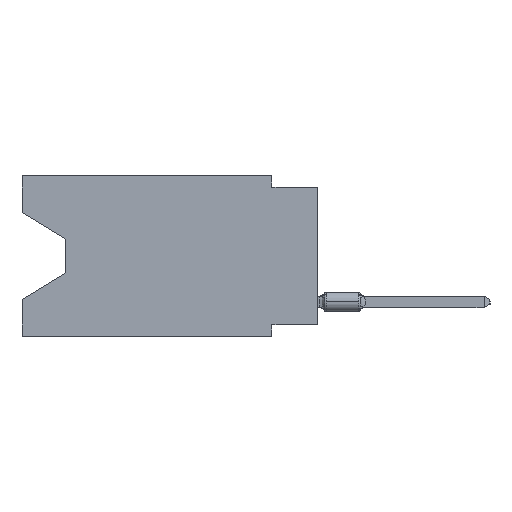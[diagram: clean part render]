
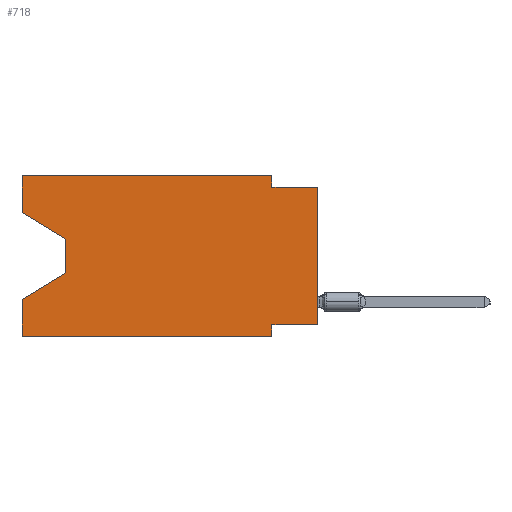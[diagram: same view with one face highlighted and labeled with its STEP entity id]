
A CAD part, left-side view. The second image highlights one B-rep face of the part: STEP entity #718.
In plain terms, the highlighted planar face has unit normal (-1, 0, 0).
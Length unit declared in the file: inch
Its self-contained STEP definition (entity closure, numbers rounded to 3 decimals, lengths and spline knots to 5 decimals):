
#529 = VERTEX_POINT ( 'NONE', #28425 ) ;
#718 = ADVANCED_FACE ( 'NONE', ( #73550 ), #9731, .F. ) ;
#1139 = EDGE_CURVE ( 'NONE', #39890, #15098, #31501, .T. ) ;
#1397 = CARTESIAN_POINT ( 'NONE',  ( 0., 0.55, -0.212 ) ) ;
#1615 = CARTESIAN_POINT ( 'NONE',  ( 0., 0.55, -0.138 ) ) ;
#1846 = VECTOR ( 'NONE', #88715, 39.37008 ) ;
#2038 = CARTESIAN_POINT ( 'NONE',  ( 0., 0.55, -0.138 ) ) ;
#2410 = LINE ( 'NONE', #39551, #10619 ) ;
#2520 = DIRECTION ( 'NONE',  ( 0., 0., -1. ) ) ;
#3393 = ORIENTED_EDGE ( 'NONE', *, *, #14539, .F. ) ;
#3409 = VERTEX_POINT ( 'NONE', #2038 ) ;
#3998 = VECTOR ( 'NONE', #41100, 39.37008 ) ;
#4539 = ORIENTED_EDGE ( 'NONE', *, *, #81420, .F. ) ;
#5720 = EDGE_CURVE ( 'NONE', #39890, #23113, #46511, .T. ) ;
#6797 = VECTOR ( 'NONE', #34415, 39.37008 ) ;
#7557 = ORIENTED_EDGE ( 'NONE', *, *, #41172, .T. ) ;
#9021 = VERTEX_POINT ( 'NONE', #71964 ) ;
#9731 = PLANE ( 'NONE',  #26192 ) ;
#10619 = VECTOR ( 'NONE', #87666, 39.37008 ) ;
#12242 = CARTESIAN_POINT ( 'NONE',  ( 0., 0.1, 0. ) ) ;
#12464 = ORIENTED_EDGE ( 'NONE', *, *, #36770, .F. ) ;
#12671 = LINE ( 'NONE', #49007, #3998 ) ;
#12762 = VERTEX_POINT ( 'NONE', #62096 ) ;
#12783 = EDGE_CURVE ( 'NONE', #80921, #50967, #25815, .T. ) ;
#13829 = VECTOR ( 'NONE', #77037, 39.37008 ) ;
#14100 = VECTOR ( 'NONE', #76528, 39.37008 ) ;
#14539 = EDGE_CURVE ( 'NONE', #50967, #12762, #84427, .T. ) ;
#15098 = VERTEX_POINT ( 'NONE', #60934 ) ;
#17013 = LINE ( 'NONE', #67295, #1846 ) ;
#17425 = CARTESIAN_POINT ( 'NONE',  ( 0., 0.645, 0. ) ) ;
#17996 = CARTESIAN_POINT ( 'NONE',  ( 0., 0.645, -0.35 ) ) ;
#19240 = VECTOR ( 'NONE', #33089, 39.37008 ) ;
#19480 = DIRECTION ( 'NONE',  ( 1., 0., 0. ) ) ;
#19535 = ORIENTED_EDGE ( 'NONE', *, *, #32777, .F. ) ;
#20206 = LINE ( 'NONE', #48613, #13829 ) ;
#22618 = EDGE_CURVE ( 'NONE', #48792, #23113, #12671, .T. ) ;
#23048 = EDGE_LOOP ( 'NONE', ( #25840, #46961, #44289, #46585, #39446, #19535, #4539, #7557, #12464, #3393, #65262, #60566 ) ) ;
#23113 = VERTEX_POINT ( 'NONE', #63306 ) ;
#25268 = CARTESIAN_POINT ( 'NONE',  ( 0., 0.1, -0.325 ) ) ;
#25815 = LINE ( 'NONE', #39312, #49817 ) ;
#25840 = ORIENTED_EDGE ( 'NONE', *, *, #50971, .T. ) ;
#26192 = AXIS2_PLACEMENT_3D ( 'NONE', #87993, #19480, #61389 ) ;
#27228 = EDGE_CURVE ( 'NONE', #66540, #80921, #61488, .T. ) ;
#28425 = CARTESIAN_POINT ( 'NONE',  ( 0., 0., -0.325 ) ) ;
#28812 = LINE ( 'NONE', #90780, #6797 ) ;
#31501 = LINE ( 'NONE', #17996, #70985 ) ;
#32777 = EDGE_CURVE ( 'NONE', #59226, #15098, #20206, .T. ) ;
#33089 = DIRECTION ( 'NONE',  ( 0., 0., 1. ) ) ;
#34415 = DIRECTION ( 'NONE',  ( 0., -1., 0. ) ) ;
#36770 = EDGE_CURVE ( 'NONE', #12762, #9021, #28812, .T. ) ;
#39312 = CARTESIAN_POINT ( 'NONE',  ( 0., 0.645, 0. ) ) ;
#39446 = ORIENTED_EDGE ( 'NONE', *, *, #1139, .T. ) ;
#39551 = CARTESIAN_POINT ( 'NONE',  ( 0., 0., -0.325 ) ) ;
#39890 = VERTEX_POINT ( 'NONE', #67906 ) ;
#41100 = DIRECTION ( 'NONE',  ( 0., 0.855, -0.519 ) ) ;
#41172 = EDGE_CURVE ( 'NONE', #529, #9021, #85745, .T. ) ;
#44289 = ORIENTED_EDGE ( 'NONE', *, *, #22618, .T. ) ;
#44481 = LINE ( 'NONE', #1615, #58556 ) ;
#44583 = DIRECTION ( 'NONE',  ( 0., -1., 0. ) ) ;
#46511 = LINE ( 'NONE', #83286, #49220 ) ;
#46585 = ORIENTED_EDGE ( 'NONE', *, *, #5720, .F. ) ;
#46961 = ORIENTED_EDGE ( 'NONE', *, *, #83944, .T. ) ;
#47075 = CARTESIAN_POINT ( 'NONE',  ( 0., 0.645, 0. ) ) ;
#48613 = CARTESIAN_POINT ( 'NONE',  ( 0., 0.1, -0.35 ) ) ;
#48792 = VERTEX_POINT ( 'NONE', #1397 ) ;
#48964 = CARTESIAN_POINT ( 'NONE',  ( 0., 0., 0. ) ) ;
#49007 = CARTESIAN_POINT ( 'NONE',  ( 0., 0.55, -0.212 ) ) ;
#49220 = VECTOR ( 'NONE', #74912, 39.37008 ) ;
#49817 = VECTOR ( 'NONE', #75630, 39.37008 ) ;
#50967 = VERTEX_POINT ( 'NONE', #58027 ) ;
#50971 = EDGE_CURVE ( 'NONE', #66540, #3409, #17013, .T. ) ;
#58027 = CARTESIAN_POINT ( 'NONE',  ( 0., 0.1, 0. ) ) ;
#58556 = VECTOR ( 'NONE', #2520, 39.37008 ) ;
#59226 = VERTEX_POINT ( 'NONE', #25268 ) ;
#60566 = ORIENTED_EDGE ( 'NONE', *, *, #27228, .F. ) ;
#60707 = VECTOR ( 'NONE', #70832, 39.37008 ) ;
#60934 = CARTESIAN_POINT ( 'NONE',  ( 0., 0.1, -0.35 ) ) ;
#61389 = DIRECTION ( 'NONE',  ( 0., 0., -1. ) ) ;
#61488 = LINE ( 'NONE', #47075, #19240 ) ;
#62096 = CARTESIAN_POINT ( 'NONE',  ( 0., 0.1, -0.025 ) ) ;
#63241 = CARTESIAN_POINT ( 'NONE',  ( 0., 0.645, -0.08025 ) ) ;
#63306 = CARTESIAN_POINT ( 'NONE',  ( 0., 0.645, -0.26975 ) ) ;
#65262 = ORIENTED_EDGE ( 'NONE', *, *, #12783, .F. ) ;
#66540 = VERTEX_POINT ( 'NONE', #63241 ) ;
#67295 = CARTESIAN_POINT ( 'NONE',  ( 0., 0.645, -0.08025 ) ) ;
#67906 = CARTESIAN_POINT ( 'NONE',  ( 0., 0.645, -0.35 ) ) ;
#70832 = DIRECTION ( 'NONE',  ( 0., 0., 1. ) ) ;
#70985 = VECTOR ( 'NONE', #44583, 39.37008 ) ;
#71964 = CARTESIAN_POINT ( 'NONE',  ( 0., 0., -0.025 ) ) ;
#73550 = FACE_OUTER_BOUND ( 'NONE', #23048, .T. ) ;
#74912 = DIRECTION ( 'NONE',  ( 0., 0., 1. ) ) ;
#75630 = DIRECTION ( 'NONE',  ( 0., -1., 0. ) ) ;
#76528 = DIRECTION ( 'NONE',  ( 0., 0., -1. ) ) ;
#77037 = DIRECTION ( 'NONE',  ( 0., 0., -1. ) ) ;
#80921 = VERTEX_POINT ( 'NONE', #17425 ) ;
#81420 = EDGE_CURVE ( 'NONE', #529, #59226, #2410, .T. ) ;
#83286 = CARTESIAN_POINT ( 'NONE',  ( 0., 0.645, 0. ) ) ;
#83944 = EDGE_CURVE ( 'NONE', #3409, #48792, #44481, .T. ) ;
#84427 = LINE ( 'NONE', #12242, #14100 ) ;
#85745 = LINE ( 'NONE', #48964, #60707 ) ;
#87666 = DIRECTION ( 'NONE',  ( 0., 1., 0. ) ) ;
#87993 = CARTESIAN_POINT ( 'NONE',  ( 0., 0.645, 0. ) ) ;
#88715 = DIRECTION ( 'NONE',  ( 0., -0.855, -0.519 ) ) ;
#90780 = CARTESIAN_POINT ( 'NONE',  ( 0., 0., -0.025 ) ) ;
